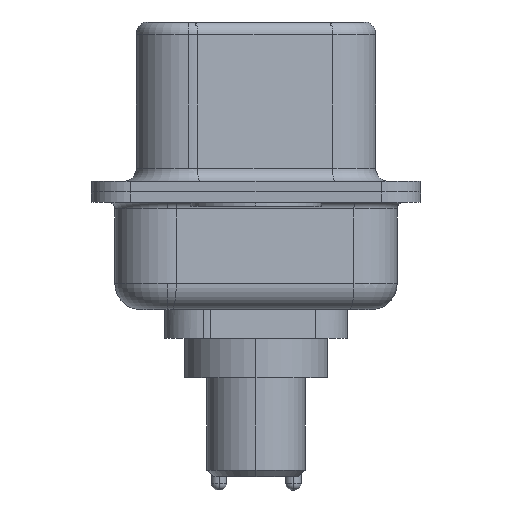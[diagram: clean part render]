
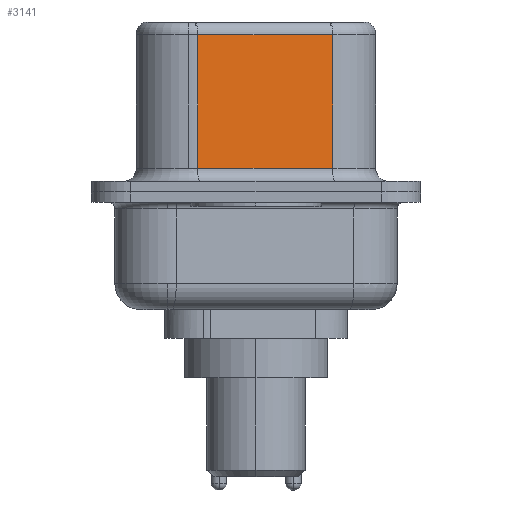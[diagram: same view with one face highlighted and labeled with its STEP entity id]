
A CAD part, left-side view. The second image highlights one B-rep face of the part: STEP entity #3141.
In plain terms, the highlighted planar face has unit normal (-0.985, -0.174, 0).
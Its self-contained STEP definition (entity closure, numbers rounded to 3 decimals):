
#501 = DIRECTION ( 'NONE',  ( 0.174, -0.985, 0. ) ) ;
#966 = LINE ( 'NONE', #19354, #12117 ) ;
#1338 = LINE ( 'NONE', #11647, #9499 ) ;
#1567 = CARTESIAN_POINT ( 'NONE',  ( 3.67, 2.233, 0.9 ) ) ;
#1598 = DIRECTION ( 'NONE',  ( -0.174, 0.985, 0. ) ) ;
#2185 = ORIENTED_EDGE ( 'NONE', *, *, #18229, .F. ) ;
#2531 = DIRECTION ( 'NONE',  ( 0., 0., -1. ) ) ;
#3141 = ADVANCED_FACE ( 'NONE', ( #17333 ), #17991, .F. ) ;
#3172 = VECTOR ( 'NONE', #501, 1000. ) ;
#3839 = VERTEX_POINT ( 'NONE', #4135 ) ;
#3919 = EDGE_LOOP ( 'NONE', ( #2185, #7741, #16090, #13660 ) ) ;
#4075 = CARTESIAN_POINT ( 'NONE',  ( 4.58, -2.927, 6.02 ) ) ;
#4135 = CARTESIAN_POINT ( 'NONE',  ( 4.58, -2.927, 6.02 ) ) ;
#5036 = VERTEX_POINT ( 'NONE', #18312 ) ;
#7250 = AXIS2_PLACEMENT_3D ( 'NONE', #14254, #16387, #1598 ) ;
#7360 = DIRECTION ( 'NONE',  ( 0., 0., -1. ) ) ;
#7741 = ORIENTED_EDGE ( 'NONE', *, *, #15924, .T. ) ;
#8980 = VECTOR ( 'NONE', #14707, 1000. ) ;
#9499 = VECTOR ( 'NONE', #2531, 1000. ) ;
#10267 = VERTEX_POINT ( 'NONE', #1567 ) ;
#10804 = LINE ( 'NONE', #17172, #3172 ) ;
#11069 = EDGE_CURVE ( 'NONE', #10267, #14832, #10804, .T. ) ;
#11647 = CARTESIAN_POINT ( 'NONE',  ( 3.67, 2.233, 6.52 ) ) ;
#12117 = VECTOR ( 'NONE', #7360, 1000. ) ;
#13660 = ORIENTED_EDGE ( 'NONE', *, *, #11069, .T. ) ;
#14254 = CARTESIAN_POINT ( 'NONE',  ( 4.58, -2.927, 6.52 ) ) ;
#14573 = LINE ( 'NONE', #4075, #8980 ) ;
#14707 = DIRECTION ( 'NONE',  ( -0.174, 0.985, 0. ) ) ;
#14832 = VERTEX_POINT ( 'NONE', #15561 ) ;
#15561 = CARTESIAN_POINT ( 'NONE',  ( 4.58, -2.927, 0.9 ) ) ;
#15903 = EDGE_CURVE ( 'NONE', #5036, #10267, #1338, .T. ) ;
#15924 = EDGE_CURVE ( 'NONE', #3839, #5036, #14573, .T. ) ;
#16090 = ORIENTED_EDGE ( 'NONE', *, *, #15903, .T. ) ;
#16387 = DIRECTION ( 'NONE',  ( 0.985, 0.174, 0. ) ) ;
#17172 = CARTESIAN_POINT ( 'NONE',  ( 4.58, -2.927, 0.9 ) ) ;
#17333 = FACE_OUTER_BOUND ( 'NONE', #3919, .T. ) ;
#17991 = PLANE ( 'NONE',  #7250 ) ;
#18229 = EDGE_CURVE ( 'NONE', #3839, #14832, #966, .T. ) ;
#18312 = CARTESIAN_POINT ( 'NONE',  ( 3.67, 2.233, 6.02 ) ) ;
#19354 = CARTESIAN_POINT ( 'NONE',  ( 4.58, -2.927, 6.52 ) ) ;
